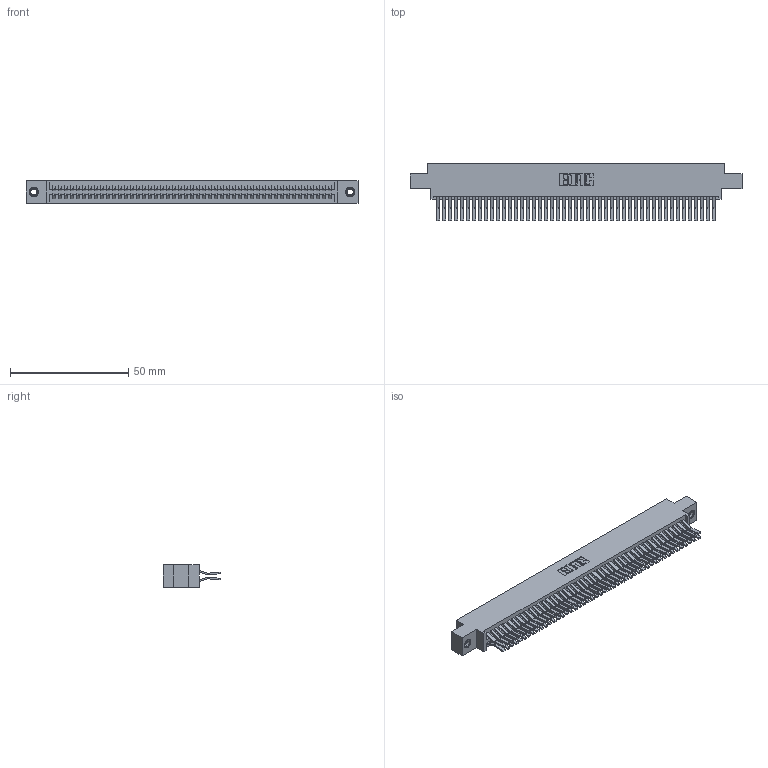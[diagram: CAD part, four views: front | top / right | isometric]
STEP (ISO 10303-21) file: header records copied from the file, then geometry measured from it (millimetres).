
FILE_DESCRIPTION (( 'STEP AP203' ), '1' );
FILE_NAME ('395-094-560-807.STEP', '2019-10-25T23:35:38', ( '' ), ( '' ), 'SwSTEP 2.0', 'SolidWorks 2016', '' );
FILE_SCHEMA (( 'CONFIG_CONTROL_DESIGN' ));
Length unit declared in the file: inch
Products named in the file (4): 345 Part_0.170 Offset - 0.156 Dia-TI; 345-292-001_560 Tail; 345-250-001_345-250-005-103; 395-094-560-807
Assembly tree (97 placements, depth 2):
  395-094-560-807
    345 Part_0.170 Offset - 0.156 Dia-TI
    345-292-001_560 Tail  x94
    345-250-001_345-250-005-103  x2
Bounding box: 140.59 x 24.45 x 9.4 mm (x, y, z)
Volume: 14192.6 mm3; surface area: 22831.9 mm2
Topology: 97 solids, 97 shells, 5078 faces, 15059 edges, 9906 vertices
Faces by surface type: plane 3218, cylinder 1844, cone 12, torus 4
Entity records: 37610 total; most frequent: CARTESIAN_POINT 6283, ORIENTED_EDGE 6210, DIRECTION 5563, EDGE_CURVE 3105, VECTOR 2761, LINE 2761, VERTEX_POINT 2064, AXIS2_PLACEMENT_3D 1401
